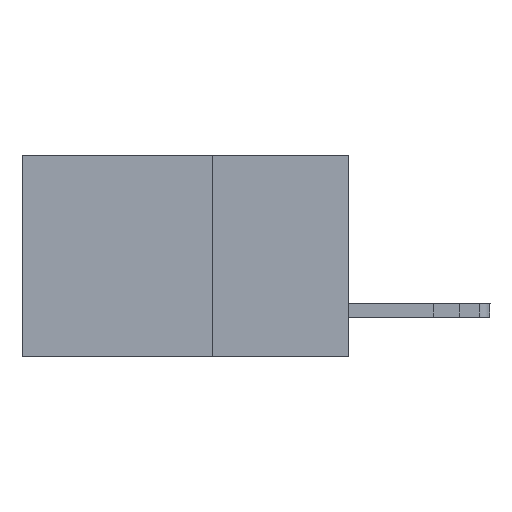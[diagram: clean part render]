
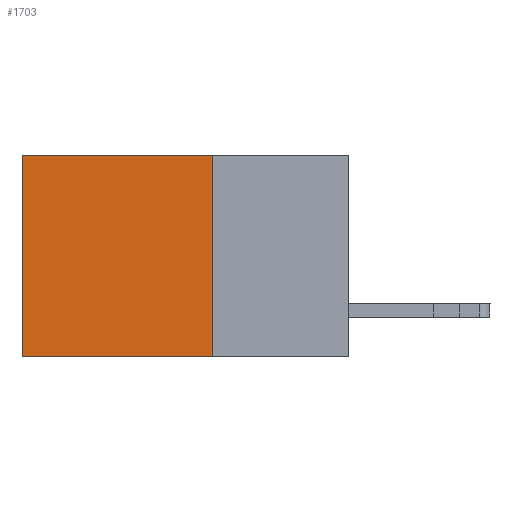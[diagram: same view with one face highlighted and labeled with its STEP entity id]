
A CAD part, left-side view. The second image highlights one B-rep face of the part: STEP entity #1703.
In plain terms, the highlighted planar face has unit normal (-1, 0, 0).
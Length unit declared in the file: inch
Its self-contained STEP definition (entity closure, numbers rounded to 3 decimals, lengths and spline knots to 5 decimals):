
#1703 = ADVANCED_FACE ( 'NONE', ( #4557 ), #8709, .F. ) ;
#1774 = LINE ( 'NONE', #4122, #8007 ) ;
#2346 = VERTEX_POINT ( 'NONE', #11533 ) ;
#4122 = CARTESIAN_POINT ( 'NONE',  ( 0.2615, 0.6, -0.37 ) ) ;
#4317 = EDGE_CURVE ( 'NONE', #15785, #6343, #6870, .T. ) ;
#4557 = FACE_OUTER_BOUND ( 'NONE', #11956, .T. ) ;
#4970 = DIRECTION ( 'NONE',  ( 0., 0., -1. ) ) ;
#5171 = ORIENTED_EDGE ( 'NONE', *, *, #6050, .T. ) ;
#5996 = VECTOR ( 'NONE', #10669, 39.37008 ) ;
#6050 = EDGE_CURVE ( 'NONE', #2346, #12830, #1774, .T. ) ;
#6218 = DIRECTION ( 'NONE',  ( 1., 0., 0. ) ) ;
#6343 = VERTEX_POINT ( 'NONE', #8349 ) ;
#6451 = AXIS2_PLACEMENT_3D ( 'NONE', #11285, #6218, #15038 ) ;
#6800 = LINE ( 'NONE', #14380, #5996 ) ;
#6870 = LINE ( 'NONE', #11329, #12824 ) ;
#7934 = CARTESIAN_POINT ( 'NONE',  ( 0.2615, 0.6, -0.37 ) ) ;
#8007 = VECTOR ( 'NONE', #14214, 39.37008 ) ;
#8349 = CARTESIAN_POINT ( 'NONE',  ( 0.2615, 0.25, -0.37 ) ) ;
#8475 = DIRECTION ( 'NONE',  ( 0., 1., 0. ) ) ;
#8532 = ORIENTED_EDGE ( 'NONE', *, *, #12502, .F. ) ;
#8709 = PLANE ( 'NONE',  #6451 ) ;
#8928 = ORIENTED_EDGE ( 'NONE', *, *, #15471, .T. ) ;
#10669 = DIRECTION ( 'NONE',  ( 0., 1., 0. ) ) ;
#11285 = CARTESIAN_POINT ( 'NONE',  ( 0.2615, 0.25, -0.37 ) ) ;
#11329 = CARTESIAN_POINT ( 'NONE',  ( 0.2615, 0.25, -0.37 ) ) ;
#11533 = CARTESIAN_POINT ( 'NONE',  ( 0.2615, 0.6, 0. ) ) ;
#11604 = VECTOR ( 'NONE', #8475, 39.37008 ) ;
#11939 = ORIENTED_EDGE ( 'NONE', *, *, #4317, .F. ) ;
#11956 = EDGE_LOOP ( 'NONE', ( #5171, #8532, #11939, #8928 ) ) ;
#12502 = EDGE_CURVE ( 'NONE', #6343, #12830, #14910, .T. ) ;
#12517 = CARTESIAN_POINT ( 'NONE',  ( 0.2615, 0.25, 0. ) ) ;
#12824 = VECTOR ( 'NONE', #4970, 39.37008 ) ;
#12830 = VERTEX_POINT ( 'NONE', #7934 ) ;
#14214 = DIRECTION ( 'NONE',  ( 0., 0., -1. ) ) ;
#14380 = CARTESIAN_POINT ( 'NONE',  ( 0.2615, 0.25, 0. ) ) ;
#14760 = CARTESIAN_POINT ( 'NONE',  ( 0.2615, 0.25, -0.37 ) ) ;
#14910 = LINE ( 'NONE', #14760, #11604 ) ;
#15038 = DIRECTION ( 'NONE',  ( 0., 0., -1. ) ) ;
#15471 = EDGE_CURVE ( 'NONE', #15785, #2346, #6800, .T. ) ;
#15785 = VERTEX_POINT ( 'NONE', #12517 ) ;
